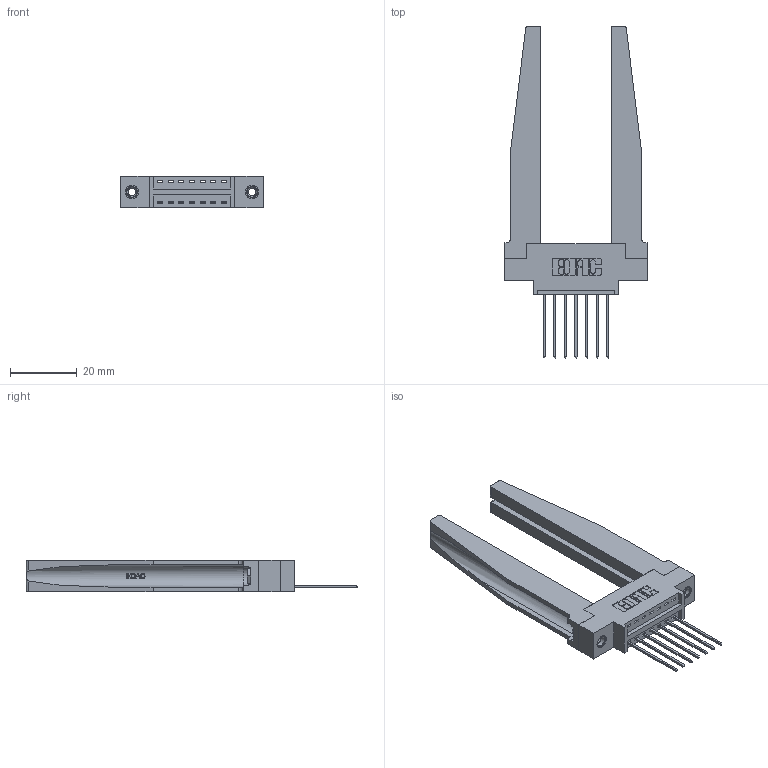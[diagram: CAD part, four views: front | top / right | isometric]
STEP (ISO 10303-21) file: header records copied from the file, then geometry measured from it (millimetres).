
FILE_DESCRIPTION (( 'STEP AP203' ), '1' );
FILE_NAME ('396-007-541-678.STEP', '2019-10-25T18:32:18', ( '' ), ( '' ), 'SwSTEP 2.0', 'SolidWorks 2016', '' );
FILE_SCHEMA (( 'CONFIG_CONTROL_DESIGN' ));
Length unit declared in the file: inch
Products named in the file (5): 345-250-001_345-250-001-102; 346 Part_0.170 Offset - 0.156 Dia-TH; 346-220-078_345-220-078; 345-292-001_345-293-141; 396-007-541-678
Assembly tree (12 placements, depth 2):
  396-007-541-678
    346 Part_0.170 Offset - 0.156 Dia-TH
    345-292-001_345-293-141  x7
    346-220-078_345-220-078  x2
    345-250-001_345-250-001-102  x2
Bounding box: 42.8 x 99.57 x 9.4 mm (x, y, z)
Volume: 10633 mm3; surface area: 11115.4 mm2
Topology: 12 solids, 12 shells, 766 faces, 2181 edges, 1434 vertices
Faces by surface type: plane 502, cylinder 212, bspline 36, cone 12, torus 4
Entity records: 13954 total; most frequent: CARTESIAN_POINT 3316, ORIENTED_EDGE 2146, DIRECTION 1953, EDGE_CURVE 1073, VECTOR 819, LINE 819, VERTEX_POINT 708, AXIS2_PLACEMENT_3D 567
